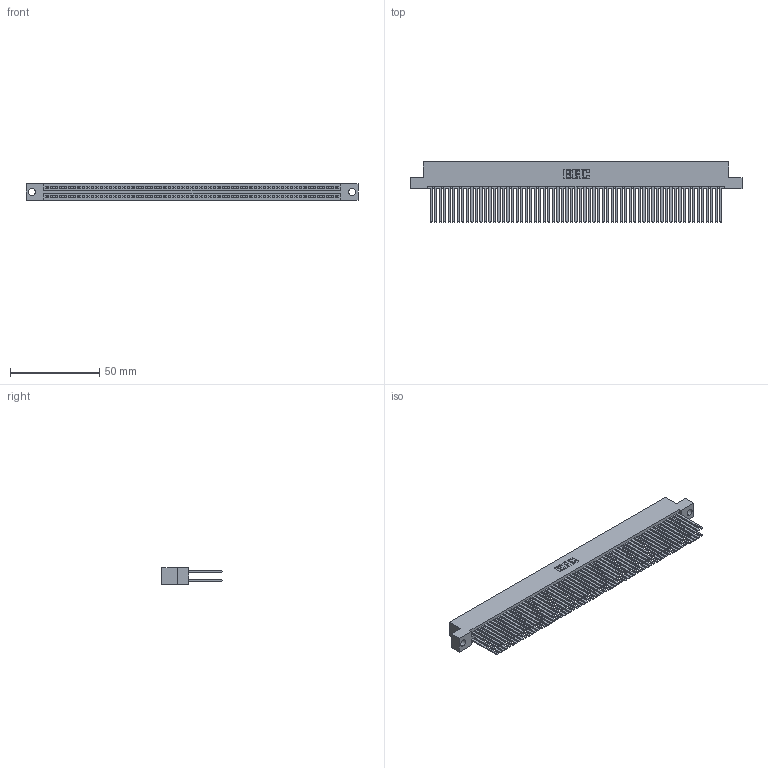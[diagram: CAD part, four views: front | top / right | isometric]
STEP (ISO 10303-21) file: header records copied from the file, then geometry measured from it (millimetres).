
FILE_DESCRIPTION (( 'STEP AP203' ), '1' );
FILE_NAME ('345-130-544-204.STEP', '2021-05-25T20:47:47', ( '' ), ( '' ), 'SwSTEP 2.0', 'SolidWorks 2020', '' );
FILE_SCHEMA (( 'CONFIG_CONTROL_DESIGN' ));
Length unit declared in the file: inch
Products named in the file (3): 345 Part_Flush Mounting Lugs - 0.156 Dia-TI; 345-130-544-204; 345-292-001_345-293-144
Assembly tree (131 placements, depth 2):
  345-130-544-204
    345 Part_Flush Mounting Lugs - 0.156 Dia-TI
    345-292-001_345-293-144  x130
Bounding box: 186.31 x 33.96 x 9.4 mm (x, y, z)
Volume: 20028.1 mm3; surface area: 35243.2 mm2
Topology: 131 solids, 131 shells, 5860 faces, 17407 edges, 11430 vertices
Faces by surface type: plane 3864, cylinder 1996
Entity records: 48139 total; most frequent: CARTESIAN_POINT 8050, ORIENTED_EDGE 7982, DIRECTION 7067, EDGE_CURVE 3991, VECTOR 3603, LINE 3603, VERTEX_POINT 2658, AXIS2_PLACEMENT_3D 1732
